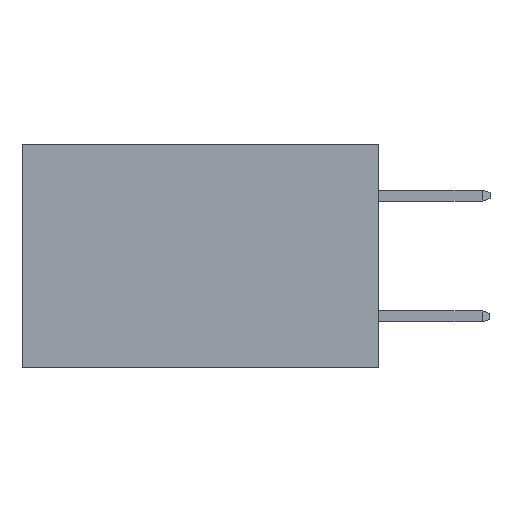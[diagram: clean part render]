
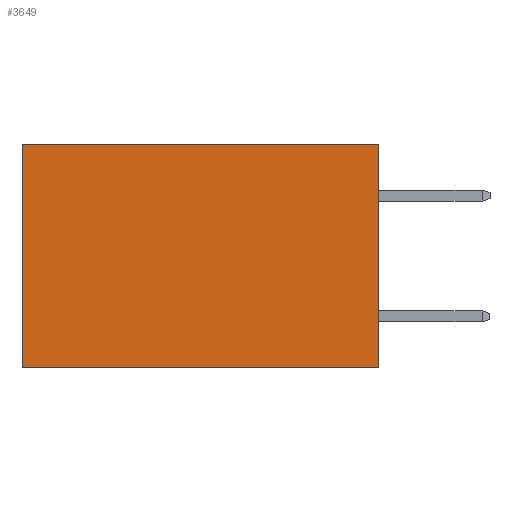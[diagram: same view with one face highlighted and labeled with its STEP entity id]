
A CAD part, left-side view. The second image highlights one B-rep face of the part: STEP entity #3649.
In plain terms, the highlighted planar face has unit normal (-1, 0, 0).
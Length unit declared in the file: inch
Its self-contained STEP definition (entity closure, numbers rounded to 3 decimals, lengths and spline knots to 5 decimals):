
#77 = EDGE_CURVE ( 'NONE', #1325, #433, #4563, .T. ) ;
#433 = VERTEX_POINT ( 'NONE', #689 ) ;
#463 = ORIENTED_EDGE ( 'NONE', *, *, #1391, .F. ) ;
#601 = VERTEX_POINT ( 'NONE', #4881 ) ;
#689 = CARTESIAN_POINT ( 'NONE',  ( 0.277, 0.59, -0.37 ) ) ;
#694 = LINE ( 'NONE', #6895, #2119 ) ;
#714 = DIRECTION ( 'NONE',  ( 0., 1., 0. ) ) ;
#780 = CARTESIAN_POINT ( 'NONE',  ( 0.277, 0., -0.37 ) ) ;
#888 = AXIS2_PLACEMENT_3D ( 'NONE', #3514, #6178, #6193 ) ;
#969 = ORIENTED_EDGE ( 'NONE', *, *, #77, .T. ) ;
#1170 = VECTOR ( 'NONE', #714, 39.37008 ) ;
#1325 = VERTEX_POINT ( 'NONE', #3978 ) ;
#1391 = EDGE_CURVE ( 'NONE', #601, #2455, #4977, .T. ) ;
#2103 = EDGE_LOOP ( 'NONE', ( #969, #5586, #463, #4053 ) ) ;
#2119 = VECTOR ( 'NONE', #4691, 39.37008 ) ;
#2124 = CARTESIAN_POINT ( 'NONE',  ( 0.277, 0., -0.37 ) ) ;
#2455 = VERTEX_POINT ( 'NONE', #3625 ) ;
#2955 = LINE ( 'NONE', #780, #1170 ) ;
#3270 = VECTOR ( 'NONE', #6197, 39.37008 ) ;
#3514 = CARTESIAN_POINT ( 'NONE',  ( 0.277, 0., -0.37 ) ) ;
#3625 = CARTESIAN_POINT ( 'NONE',  ( 0.277, 0., -0.37 ) ) ;
#3649 = ADVANCED_FACE ( 'NONE', ( #5358 ), #5764, .F. ) ;
#3978 = CARTESIAN_POINT ( 'NONE',  ( 0.277, 0.59, 0. ) ) ;
#4053 = ORIENTED_EDGE ( 'NONE', *, *, #7554, .T. ) ;
#4336 = DIRECTION ( 'NONE',  ( 0., 0., -1. ) ) ;
#4563 = LINE ( 'NONE', #5025, #5523 ) ;
#4691 = DIRECTION ( 'NONE',  ( 0., 1., 0. ) ) ;
#4881 = CARTESIAN_POINT ( 'NONE',  ( 0.277, 0., 0. ) ) ;
#4977 = LINE ( 'NONE', #2124, #3270 ) ;
#5025 = CARTESIAN_POINT ( 'NONE',  ( 0.277, 0.59, -0.37 ) ) ;
#5358 = FACE_OUTER_BOUND ( 'NONE', #2103, .T. ) ;
#5523 = VECTOR ( 'NONE', #4336, 39.37008 ) ;
#5586 = ORIENTED_EDGE ( 'NONE', *, *, #6680, .F. ) ;
#5764 = PLANE ( 'NONE',  #888 ) ;
#6178 = DIRECTION ( 'NONE',  ( 1., 0., 0. ) ) ;
#6193 = DIRECTION ( 'NONE',  ( 0., 0., -1. ) ) ;
#6197 = DIRECTION ( 'NONE',  ( 0., 0., -1. ) ) ;
#6680 = EDGE_CURVE ( 'NONE', #2455, #433, #2955, .T. ) ;
#6895 = CARTESIAN_POINT ( 'NONE',  ( 0.277, 0., 0. ) ) ;
#7554 = EDGE_CURVE ( 'NONE', #601, #1325, #694, .T. ) ;
